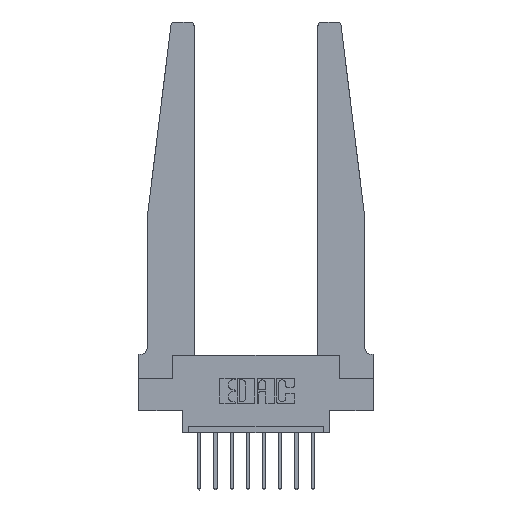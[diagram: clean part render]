
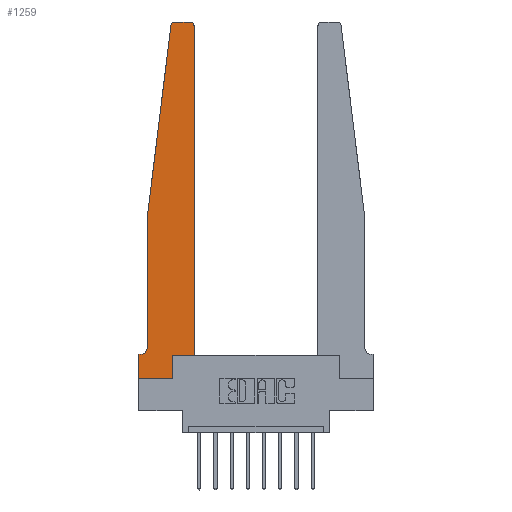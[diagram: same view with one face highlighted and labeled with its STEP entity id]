
A CAD part, top view. The second image highlights one B-rep face of the part: STEP entity #1259.
In plain terms, the highlighted planar face has unit normal (0, 0, 1).
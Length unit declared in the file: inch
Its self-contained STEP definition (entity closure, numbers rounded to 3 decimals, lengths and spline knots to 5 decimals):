
#62 = VERTEX_POINT ( 'NONE', #13887 ) ;
#186 = VERTEX_POINT ( 'NONE', #1358 ) ;
#195 = DIRECTION ( 'NONE',  ( 1., 0., 0. ) ) ;
#229 = VERTEX_POINT ( 'NONE', #9336 ) ;
#278 = EDGE_CURVE ( 'NONE', #2830, #12993, #9530, .T. ) ;
#579 = ORIENTED_EDGE ( 'NONE', *, *, #11802, .T. ) ;
#756 = ORIENTED_EDGE ( 'NONE', *, *, #1096, .T. ) ;
#977 = DIRECTION ( 'NONE',  ( 0., 0., -1. ) ) ;
#1096 = EDGE_CURVE ( 'NONE', #11137, #229, #6036, .T. ) ;
#1259 = ADVANCED_FACE ( 'NONE', ( #12624 ), #7986, .T. ) ;
#1358 = CARTESIAN_POINT ( 'NONE',  ( 0.395, 2.75, 0.37 ) ) ;
#2037 = CARTESIAN_POINT ( 'NONE',  ( 0.27653, 2.75, 0.37 ) ) ;
#2102 = DIRECTION ( 'NONE',  ( -1., 0., 0. ) ) ;
#2154 = VECTOR ( 'NONE', #11572, 39.37008 ) ;
#2363 = ORIENTED_EDGE ( 'NONE', *, *, #7320, .T. ) ;
#2596 = DIRECTION ( 'NONE',  ( -1., 0., 0. ) ) ;
#2642 = EDGE_LOOP ( 'NONE', ( #10052, #2729, #7771, #5178, #8907, #4547, #9603, #9354, #4977, #756, #579, #2363 ) ) ;
#2729 = ORIENTED_EDGE ( 'NONE', *, *, #278, .T. ) ;
#2830 = VERTEX_POINT ( 'NONE', #2037 ) ;
#2930 = LINE ( 'NONE', #7663, #6419 ) ;
#3113 = VECTOR ( 'NONE', #2596, 39.37008 ) ;
#3224 = VERTEX_POINT ( 'NONE', #9821 ) ;
#3468 = LINE ( 'NONE', #9137, #3113 ) ;
#3593 = LINE ( 'NONE', #11672, #2154 ) ;
#3779 = VERTEX_POINT ( 'NONE', #9951 ) ;
#4081 = CARTESIAN_POINT ( 'NONE',  ( 0.065, 1.25, 0.37 ) ) ;
#4100 = CARTESIAN_POINT ( 'NONE',  ( 0.2605, 0.18, 0.37 ) ) ;
#4202 = CARTESIAN_POINT ( 'NONE',  ( 0.395, 2.72, 0.37 ) ) ;
#4389 = LINE ( 'NONE', #9721, #13751 ) ;
#4541 = EDGE_CURVE ( 'NONE', #6911, #11137, #8523, .T. ) ;
#4547 = ORIENTED_EDGE ( 'NONE', *, *, #6147, .T. ) ;
#4761 = AXIS2_PLACEMENT_3D ( 'NONE', #10031, #8860, #11279 ) ;
#4977 = ORIENTED_EDGE ( 'NONE', *, *, #4541, .T. ) ;
#5075 = EDGE_CURVE ( 'NONE', #6322, #62, #7969, .T. ) ;
#5178 = ORIENTED_EDGE ( 'NONE', *, *, #5075, .T. ) ;
#5225 = AXIS2_PLACEMENT_3D ( 'NONE', #5829, #6937, #195 ) ;
#5321 = DIRECTION ( 'NONE',  ( 1., 0., 0. ) ) ;
#5360 = CARTESIAN_POINT ( 'NONE',  ( 0.015, 0.2375, 0.37 ) ) ;
#5829 = CARTESIAN_POINT ( 'NONE',  ( 0., 0.1875, 0.37 ) ) ;
#5908 = DIRECTION ( 'NONE',  ( 0., -1., 0. ) ) ;
#6036 = LINE ( 'NONE', #9826, #11576 ) ;
#6046 = VECTOR ( 'NONE', #8514, 39.37008 ) ;
#6048 = LINE ( 'NONE', #13349, #12124 ) ;
#6147 = EDGE_CURVE ( 'NONE', #3224, #3779, #6048, .T. ) ;
#6238 = DIRECTION ( 'NONE',  ( 0., 1., 0. ) ) ;
#6322 = VERTEX_POINT ( 'NONE', #4081 ) ;
#6419 = VECTOR ( 'NONE', #13242, 39.37008 ) ;
#6421 = DIRECTION ( 'NONE',  ( 1., 0., 0. ) ) ;
#6537 = CARTESIAN_POINT ( 'NONE',  ( 0.2605, 0., 0.37 ) ) ;
#6556 = CARTESIAN_POINT ( 'NONE',  ( 0., 0., 0.37 ) ) ;
#6911 = VERTEX_POINT ( 'NONE', #6537 ) ;
#6937 = DIRECTION ( 'NONE',  ( 0., 0., 1. ) ) ;
#7107 = VECTOR ( 'NONE', #5908, 39.37008 ) ;
#7320 = EDGE_CURVE ( 'NONE', #9076, #186, #8556, .T. ) ;
#7439 = DIRECTION ( 'NONE',  ( -1., 0., 0. ) ) ;
#7663 = CARTESIAN_POINT ( 'NONE',  ( 0., 0., 0.37 ) ) ;
#7771 = ORIENTED_EDGE ( 'NONE', *, *, #13722, .T. ) ;
#7969 = LINE ( 'NONE', #12395, #7107 ) ;
#7986 = PLANE ( 'NONE',  #5225 ) ;
#8123 = AXIS2_PLACEMENT_3D ( 'NONE', #4202, #11861, #5321 ) ;
#8225 = EDGE_CURVE ( 'NONE', #10999, #6911, #4389, .T. ) ;
#8514 = DIRECTION ( 'NONE',  ( -0.122, -0.992, 0. ) ) ;
#8523 = LINE ( 'NONE', #4100, #13730 ) ;
#8556 = CIRCLE ( 'NONE', #8123, 0.03 ) ;
#8860 = DIRECTION ( 'NONE',  ( 0., 0., 1. ) ) ;
#8907 = ORIENTED_EDGE ( 'NONE', *, *, #9818, .T. ) ;
#8988 = DIRECTION ( 'NONE',  ( 1., 0., 0. ) ) ;
#9076 = VERTEX_POINT ( 'NONE', #10231 ) ;
#9137 = CARTESIAN_POINT ( 'NONE',  ( 0.25, 2.75, 0.37 ) ) ;
#9327 = EDGE_CURVE ( 'NONE', #186, #2830, #3468, .T. ) ;
#9336 = CARTESIAN_POINT ( 'NONE',  ( 0.425, 0.18, 0.37 ) ) ;
#9354 = ORIENTED_EDGE ( 'NONE', *, *, #8225, .T. ) ;
#9372 = CIRCLE ( 'NONE', #11886, 0.05 ) ;
#9530 = CIRCLE ( 'NONE', #4761, 0.03 ) ;
#9603 = ORIENTED_EDGE ( 'NONE', *, *, #9836, .T. ) ;
#9721 = CARTESIAN_POINT ( 'NONE',  ( 0., 0., 0.37 ) ) ;
#9818 = EDGE_CURVE ( 'NONE', #62, #3224, #9372, .T. ) ;
#9821 = CARTESIAN_POINT ( 'NONE',  ( 0.015, 0.1875, 0.37 ) ) ;
#9826 = CARTESIAN_POINT ( 'NONE',  ( 0.425, 0.18, 0.37 ) ) ;
#9836 = EDGE_CURVE ( 'NONE', #3779, #10999, #2930, .T. ) ;
#9951 = CARTESIAN_POINT ( 'NONE',  ( 0., 0.1875, 0.37 ) ) ;
#10031 = CARTESIAN_POINT ( 'NONE',  ( 0.27653, 2.72, 0.37 ) ) ;
#10052 = ORIENTED_EDGE ( 'NONE', *, *, #9327, .T. ) ;
#10231 = CARTESIAN_POINT ( 'NONE',  ( 0.425, 2.72, 0.37 ) ) ;
#10999 = VERTEX_POINT ( 'NONE', #6556 ) ;
#11137 = VERTEX_POINT ( 'NONE', #11162 ) ;
#11162 = CARTESIAN_POINT ( 'NONE',  ( 0.2605, 0.18, 0.37 ) ) ;
#11279 = DIRECTION ( 'NONE',  ( 1., 0., 0. ) ) ;
#11572 = DIRECTION ( 'NONE',  ( 0., 1., 0. ) ) ;
#11576 = VECTOR ( 'NONE', #8988, 39.37008 ) ;
#11672 = CARTESIAN_POINT ( 'NONE',  ( 0.425, 0.18, 0.37 ) ) ;
#11712 = CARTESIAN_POINT ( 'NONE',  ( 0.065, 1.25, 0.37 ) ) ;
#11787 = LINE ( 'NONE', #11712, #6046 ) ;
#11802 = EDGE_CURVE ( 'NONE', #229, #9076, #3593, .T. ) ;
#11861 = DIRECTION ( 'NONE',  ( 0., 0., 1. ) ) ;
#11886 = AXIS2_PLACEMENT_3D ( 'NONE', #5360, #977, #2102 ) ;
#12124 = VECTOR ( 'NONE', #7439, 39.37008 ) ;
#12395 = CARTESIAN_POINT ( 'NONE',  ( 0.065, 1.25, 0.37 ) ) ;
#12624 = FACE_OUTER_BOUND ( 'NONE', #2642, .T. ) ;
#12985 = CARTESIAN_POINT ( 'NONE',  ( 0.24675, 2.72367, 0.37 ) ) ;
#12993 = VERTEX_POINT ( 'NONE', #12985 ) ;
#13242 = DIRECTION ( 'NONE',  ( 0., -1., 0. ) ) ;
#13349 = CARTESIAN_POINT ( 'NONE',  ( 0.065, 0.1875, 0.37 ) ) ;
#13722 = EDGE_CURVE ( 'NONE', #12993, #6322, #11787, .T. ) ;
#13730 = VECTOR ( 'NONE', #6238, 39.37008 ) ;
#13751 = VECTOR ( 'NONE', #6421, 39.37008 ) ;
#13887 = CARTESIAN_POINT ( 'NONE',  ( 0.065, 0.2375, 0.37 ) ) ;
